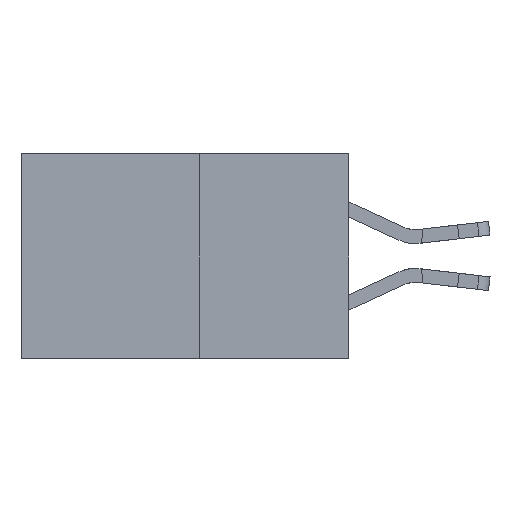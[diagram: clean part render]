
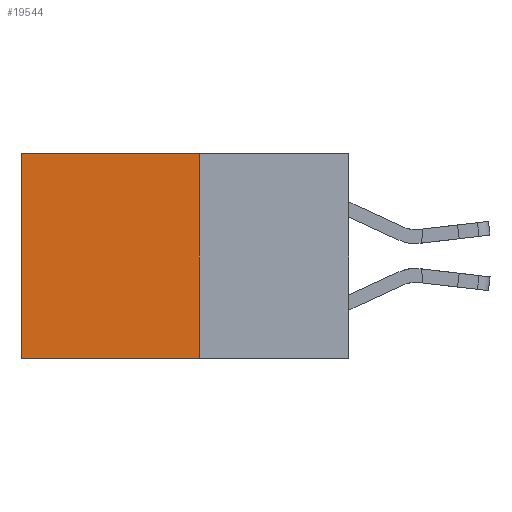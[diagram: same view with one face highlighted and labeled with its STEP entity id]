
A CAD part, left-side view. The second image highlights one B-rep face of the part: STEP entity #19544.
In plain terms, the highlighted planar face has unit normal (-1, 0, 0).
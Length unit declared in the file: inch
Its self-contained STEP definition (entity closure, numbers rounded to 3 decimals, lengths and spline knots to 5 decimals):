
#372 = VECTOR ( 'NONE', #11010, 39.37008 ) ;
#1151 = VECTOR ( 'NONE', #15467, 39.37008 ) ;
#1500 = EDGE_CURVE ( 'NONE', #6324, #19555, #9999, .T. ) ;
#2818 = EDGE_LOOP ( 'NONE', ( #17978, #15247, #14890, #17389 ) ) ;
#3465 = CARTESIAN_POINT ( 'NONE',  ( 0.277, 0.59, -0.37 ) ) ;
#3923 = EDGE_CURVE ( 'NONE', #6324, #7544, #14308, .T. ) ;
#4781 = VECTOR ( 'NONE', #7219, 39.37008 ) ;
#5340 = CARTESIAN_POINT ( 'NONE',  ( 0.277, 0.27, -0.37 ) ) ;
#6005 = LINE ( 'NONE', #10258, #1151 ) ;
#6164 = FACE_OUTER_BOUND ( 'NONE', #2818, .T. ) ;
#6324 = VERTEX_POINT ( 'NONE', #11807 ) ;
#6769 = CARTESIAN_POINT ( 'NONE',  ( 0.277, 0.27, -0.37 ) ) ;
#7219 = DIRECTION ( 'NONE',  ( 0., 0., -1. ) ) ;
#7257 = CARTESIAN_POINT ( 'NONE',  ( 0.277, 0.59, -0.37 ) ) ;
#7544 = VERTEX_POINT ( 'NONE', #9495 ) ;
#8429 = VERTEX_POINT ( 'NONE', #7257 ) ;
#8562 = DIRECTION ( 'NONE',  ( 1., 0., 0. ) ) ;
#9495 = CARTESIAN_POINT ( 'NONE',  ( 0.277, 0.27, -0.37 ) ) ;
#9880 = DIRECTION ( 'NONE',  ( 0., 0., -1. ) ) ;
#9999 = LINE ( 'NONE', #20336, #372 ) ;
#10258 = CARTESIAN_POINT ( 'NONE',  ( 0.277, 0.27, -0.37 ) ) ;
#10261 = VECTOR ( 'NONE', #9880, 39.37008 ) ;
#11010 = DIRECTION ( 'NONE',  ( 0., 1., 0. ) ) ;
#11807 = CARTESIAN_POINT ( 'NONE',  ( 0.277, 0.27, 0. ) ) ;
#14177 = LINE ( 'NONE', #3465, #4781 ) ;
#14308 = LINE ( 'NONE', #5340, #10261 ) ;
#14890 = ORIENTED_EDGE ( 'NONE', *, *, #3923, .F. ) ;
#15064 = EDGE_CURVE ( 'NONE', #7544, #8429, #6005, .T. ) ;
#15165 = AXIS2_PLACEMENT_3D ( 'NONE', #6769, #8562, #20585 ) ;
#15247 = ORIENTED_EDGE ( 'NONE', *, *, #15064, .F. ) ;
#15467 = DIRECTION ( 'NONE',  ( 0., 1., 0. ) ) ;
#17159 = PLANE ( 'NONE',  #15165 ) ;
#17389 = ORIENTED_EDGE ( 'NONE', *, *, #1500, .T. ) ;
#17742 = EDGE_CURVE ( 'NONE', #19555, #8429, #14177, .T. ) ;
#17978 = ORIENTED_EDGE ( 'NONE', *, *, #17742, .T. ) ;
#18903 = CARTESIAN_POINT ( 'NONE',  ( 0.277, 0.59, 0. ) ) ;
#19544 = ADVANCED_FACE ( 'NONE', ( #6164 ), #17159, .F. ) ;
#19555 = VERTEX_POINT ( 'NONE', #18903 ) ;
#20336 = CARTESIAN_POINT ( 'NONE',  ( 0.277, 0.27, 0. ) ) ;
#20585 = DIRECTION ( 'NONE',  ( 0., 0., -1. ) ) ;
